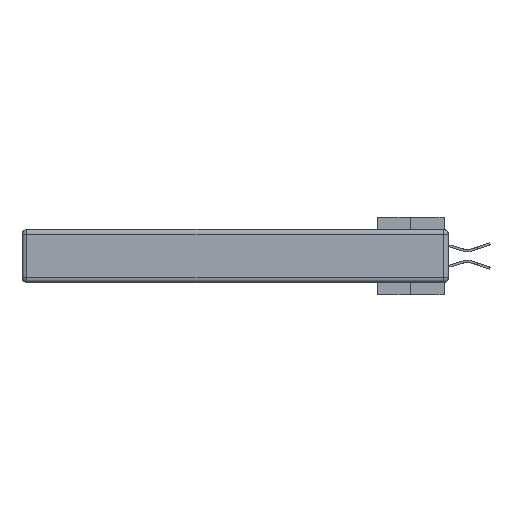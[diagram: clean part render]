
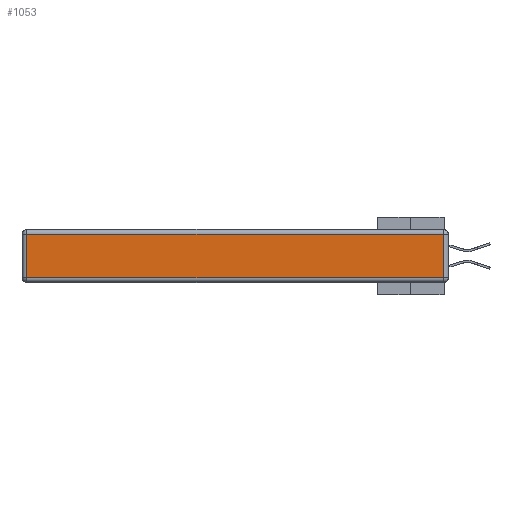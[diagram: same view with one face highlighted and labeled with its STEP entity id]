
A CAD part, left-side view. The second image highlights one B-rep face of the part: STEP entity #1053.
In plain terms, the highlighted planar face has unit normal (-1, 0, 0).
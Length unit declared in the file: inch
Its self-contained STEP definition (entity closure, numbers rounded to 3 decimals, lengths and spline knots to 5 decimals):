
#373 = DIRECTION ( 'NONE',  ( 0., 0., -1. ) ) ;
#1053 = ADVANCED_FACE ( 'NONE', ( #23508 ), #2286, .T. ) ;
#1677 = DIRECTION ( 'NONE',  ( 0., 1., 0. ) ) ;
#2283 = CARTESIAN_POINT ( 'NONE',  ( 0., 0.03, -0.343 ) ) ;
#2286 = PLANE ( 'NONE',  #22250 ) ;
#4578 = CARTESIAN_POINT ( 'NONE',  ( 0., 2.75, -0.03 ) ) ;
#4839 = EDGE_LOOP ( 'NONE', ( #18497, #8159, #15066, #30915 ) ) ;
#5315 = CARTESIAN_POINT ( 'NONE',  ( 0., 0.03, -0.313 ) ) ;
#6591 = VECTOR ( 'NONE', #26813, 39.37008 ) ;
#7255 = VERTEX_POINT ( 'NONE', #5315 ) ;
#8159 = ORIENTED_EDGE ( 'NONE', *, *, #16390, .T. ) ;
#10245 = EDGE_CURVE ( 'NONE', #13476, #12672, #32246, .T. ) ;
#12369 = CARTESIAN_POINT ( 'NONE',  ( 0., 2.72, -0.343 ) ) ;
#12672 = VERTEX_POINT ( 'NONE', #27245 ) ;
#12823 = LINE ( 'NONE', #4578, #28998 ) ;
#13476 = VERTEX_POINT ( 'NONE', #28252 ) ;
#14492 = EDGE_CURVE ( 'NONE', #12672, #7255, #16237, .T. ) ;
#14948 = EDGE_CURVE ( 'NONE', #21824, #13476, #12823, .T. ) ;
#15066 = ORIENTED_EDGE ( 'NONE', *, *, #14948, .T. ) ;
#16237 = LINE ( 'NONE', #26617, #29526 ) ;
#16390 = EDGE_CURVE ( 'NONE', #7255, #21824, #32141, .T. ) ;
#17378 = CARTESIAN_POINT ( 'NONE',  ( 0., 0., -0.343 ) ) ;
#18497 = ORIENTED_EDGE ( 'NONE', *, *, #14492, .T. ) ;
#20062 = CARTESIAN_POINT ( 'NONE',  ( 0., 0.03, -0.03 ) ) ;
#20450 = VECTOR ( 'NONE', #373, 39.37008 ) ;
#21824 = VERTEX_POINT ( 'NONE', #20062 ) ;
#22250 = AXIS2_PLACEMENT_3D ( 'NONE', #17378, #35932, #38606 ) ;
#23508 = FACE_OUTER_BOUND ( 'NONE', #4839, .T. ) ;
#26617 = CARTESIAN_POINT ( 'NONE',  ( 0., 0., -0.313 ) ) ;
#26813 = DIRECTION ( 'NONE',  ( 0., 0., 1. ) ) ;
#27245 = CARTESIAN_POINT ( 'NONE',  ( 0., 2.72, -0.313 ) ) ;
#28252 = CARTESIAN_POINT ( 'NONE',  ( 0., 2.72, -0.03 ) ) ;
#28998 = VECTOR ( 'NONE', #1677, 39.37008 ) ;
#29526 = VECTOR ( 'NONE', #35728, 39.37008 ) ;
#30915 = ORIENTED_EDGE ( 'NONE', *, *, #10245, .T. ) ;
#32141 = LINE ( 'NONE', #2283, #6591 ) ;
#32246 = LINE ( 'NONE', #12369, #20450 ) ;
#35728 = DIRECTION ( 'NONE',  ( 0., -1., 0. ) ) ;
#35932 = DIRECTION ( 'NONE',  ( -1., 0., 0. ) ) ;
#38606 = DIRECTION ( 'NONE',  ( 0., 0., 1. ) ) ;
